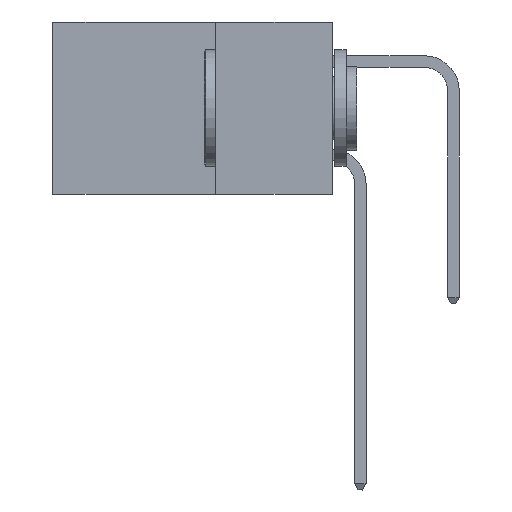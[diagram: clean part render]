
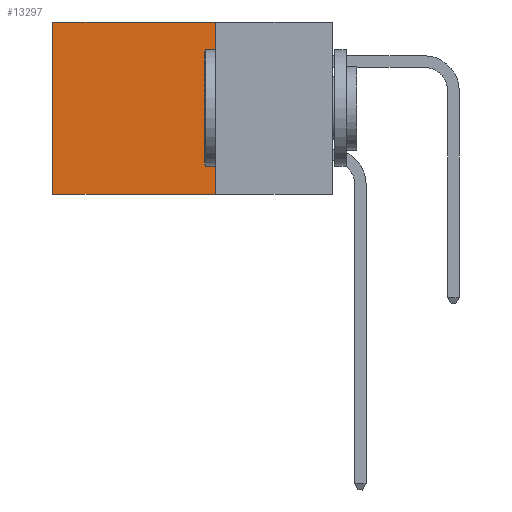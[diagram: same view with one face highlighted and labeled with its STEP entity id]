
A CAD part, left-side view. The second image highlights one B-rep face of the part: STEP entity #13297.
In plain terms, the highlighted planar face has unit normal (-1, 0, 0).
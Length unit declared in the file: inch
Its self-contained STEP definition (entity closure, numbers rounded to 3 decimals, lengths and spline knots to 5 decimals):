
#47 = LINE ( 'NONE', #5314, #7138 ) ;
#229 = VECTOR ( 'NONE', #4456, 39.37008 ) ;
#1064 = DIRECTION ( 'NONE',  ( 0., 0., -1. ) ) ;
#1666 = ORIENTED_EDGE ( 'NONE', *, *, #5210, .T. ) ;
#2713 = VERTEX_POINT ( 'NONE', #22425 ) ;
#4456 = DIRECTION ( 'NONE',  ( 0., 1., 0. ) ) ;
#4933 = ORIENTED_EDGE ( 'NONE', *, *, #13870, .F. ) ;
#5210 = EDGE_CURVE ( 'NONE', #21640, #13704, #47, .T. ) ;
#5222 = ORIENTED_EDGE ( 'NONE', *, *, #27241, .T. ) ;
#5314 = CARTESIAN_POINT ( 'NONE',  ( 0.298, 0.6, 0. ) ) ;
#6762 = ORIENTED_EDGE ( 'NONE', *, *, #15014, .F. ) ;
#7138 = VECTOR ( 'NONE', #1064, 39.37008 ) ;
#9534 = FACE_OUTER_BOUND ( 'NONE', #24954, .T. ) ;
#10148 = DIRECTION ( 'NONE',  ( 1., 0., 0. ) ) ;
#11307 = AXIS2_PLACEMENT_3D ( 'NONE', #23046, #10148, #14376 ) ;
#13297 = ADVANCED_FACE ( 'NONE', ( #9534 ), #20778, .F. ) ;
#13704 = VERTEX_POINT ( 'NONE', #26738 ) ;
#13870 = EDGE_CURVE ( 'NONE', #2713, #16746, #26686, .T. ) ;
#14144 = CARTESIAN_POINT ( 'NONE',  ( 0.298, 0.25, -0.37 ) ) ;
#14376 = DIRECTION ( 'NONE',  ( 0., 0., -1. ) ) ;
#15014 = EDGE_CURVE ( 'NONE', #16746, #13704, #26968, .T. ) ;
#16746 = VERTEX_POINT ( 'NONE', #22096 ) ;
#17692 = CARTESIAN_POINT ( 'NONE',  ( 0.298, 0.6, 0. ) ) ;
#20778 = PLANE ( 'NONE',  #11307 ) ;
#21640 = VERTEX_POINT ( 'NONE', #17692 ) ;
#21986 = VECTOR ( 'NONE', #25950, 39.37008 ) ;
#22096 = CARTESIAN_POINT ( 'NONE',  ( 0.298, 0.25, -0.37 ) ) ;
#22425 = CARTESIAN_POINT ( 'NONE',  ( 0.298, 0.25, 0. ) ) ;
#22859 = LINE ( 'NONE', #26154, #229 ) ;
#22951 = VECTOR ( 'NONE', #25225, 39.37008 ) ;
#23046 = CARTESIAN_POINT ( 'NONE',  ( 0.298, 0.25, 0. ) ) ;
#24954 = EDGE_LOOP ( 'NONE', ( #1666, #6762, #4933, #5222 ) ) ;
#25225 = DIRECTION ( 'NONE',  ( 0., 1., 0. ) ) ;
#25402 = CARTESIAN_POINT ( 'NONE',  ( 0.298, 0.25, 0. ) ) ;
#25950 = DIRECTION ( 'NONE',  ( 0., 0., -1. ) ) ;
#26154 = CARTESIAN_POINT ( 'NONE',  ( 0.298, 0.25, 0. ) ) ;
#26686 = LINE ( 'NONE', #25402, #21986 ) ;
#26738 = CARTESIAN_POINT ( 'NONE',  ( 0.298, 0.6, -0.37 ) ) ;
#26968 = LINE ( 'NONE', #14144, #22951 ) ;
#27241 = EDGE_CURVE ( 'NONE', #2713, #21640, #22859, .T. ) ;
